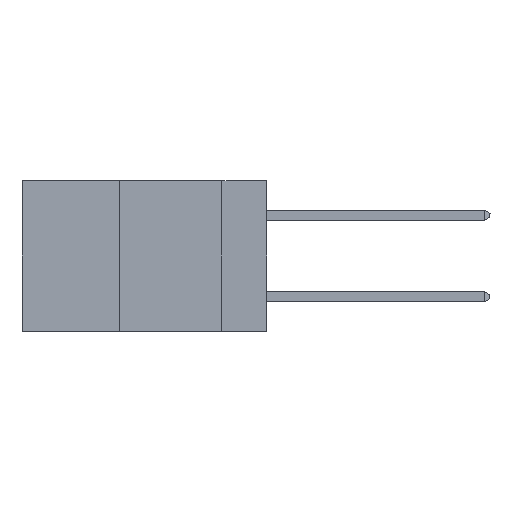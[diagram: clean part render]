
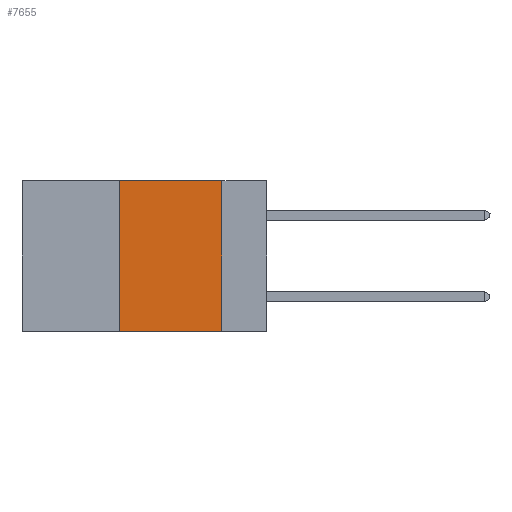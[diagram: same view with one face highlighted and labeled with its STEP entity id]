
A CAD part, left-side view. The second image highlights one B-rep face of the part: STEP entity #7655.
In plain terms, the highlighted planar face has unit normal (-1, 0, 0).
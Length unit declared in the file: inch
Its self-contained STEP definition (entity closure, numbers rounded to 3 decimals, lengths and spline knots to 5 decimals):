
#302 = LINE ( 'NONE', #19538, #10759 ) ;
#681 = PLANE ( 'NONE',  #7395 ) ;
#1203 = EDGE_CURVE ( 'NONE', #21719, #1650, #18108, .T. ) ;
#1267 = CARTESIAN_POINT ( 'NONE',  ( 0., 0.6, -0.37 ) ) ;
#1316 = VECTOR ( 'NONE', #17362, 39.37008 ) ;
#1650 = VERTEX_POINT ( 'NONE', #8465 ) ;
#2507 = DIRECTION ( 'NONE',  ( 1., 0., 0. ) ) ;
#2869 = DIRECTION ( 'NONE',  ( 0., -1., 0. ) ) ;
#3205 = LINE ( 'NONE', #1267, #8802 ) ;
#4940 = VECTOR ( 'NONE', #6041, 39.37008 ) ;
#5548 = DIRECTION ( 'NONE',  ( 0., 0., 1. ) ) ;
#6041 = DIRECTION ( 'NONE',  ( 0., 0., -1. ) ) ;
#6536 = EDGE_CURVE ( 'NONE', #13999, #1650, #3205, .T. ) ;
#6560 = ORIENTED_EDGE ( 'NONE', *, *, #6536, .T. ) ;
#6569 = ORIENTED_EDGE ( 'NONE', *, *, #14269, .F. ) ;
#7348 = CARTESIAN_POINT ( 'NONE',  ( 0., 0.11, 0. ) ) ;
#7395 = AXIS2_PLACEMENT_3D ( 'NONE', #21307, #2507, #7962 ) ;
#7655 = ADVANCED_FACE ( 'NONE', ( #18112 ), #681, .F. ) ;
#7962 = DIRECTION ( 'NONE',  ( 0., 0., -1. ) ) ;
#8093 = ORIENTED_EDGE ( 'NONE', *, *, #1203, .F. ) ;
#8243 = ORIENTED_EDGE ( 'NONE', *, *, #14006, .F. ) ;
#8465 = CARTESIAN_POINT ( 'NONE',  ( 0., 0.11, -0.37 ) ) ;
#8799 = CARTESIAN_POINT ( 'NONE',  ( 0., 0.6, 0. ) ) ;
#8802 = VECTOR ( 'NONE', #2869, 39.37008 ) ;
#9215 = CARTESIAN_POINT ( 'NONE',  ( 0., 0.11, 0. ) ) ;
#9506 = VERTEX_POINT ( 'NONE', #21395 ) ;
#10759 = VECTOR ( 'NONE', #5548, 39.37008 ) ;
#13999 = VERTEX_POINT ( 'NONE', #18053 ) ;
#14006 = EDGE_CURVE ( 'NONE', #13999, #9506, #302, .T. ) ;
#14269 = EDGE_CURVE ( 'NONE', #9506, #21719, #20765, .T. ) ;
#16131 = EDGE_LOOP ( 'NONE', ( #8093, #6569, #8243, #6560 ) ) ;
#17362 = DIRECTION ( 'NONE',  ( 0., -1., 0. ) ) ;
#18053 = CARTESIAN_POINT ( 'NONE',  ( 0., 0.36, -0.37 ) ) ;
#18108 = LINE ( 'NONE', #9215, #4940 ) ;
#18112 = FACE_OUTER_BOUND ( 'NONE', #16131, .T. ) ;
#19538 = CARTESIAN_POINT ( 'NONE',  ( 0., 0.36, 0. ) ) ;
#20765 = LINE ( 'NONE', #8799, #1316 ) ;
#21307 = CARTESIAN_POINT ( 'NONE',  ( 0., 0.6, 0. ) ) ;
#21395 = CARTESIAN_POINT ( 'NONE',  ( 0., 0.36, 0. ) ) ;
#21719 = VERTEX_POINT ( 'NONE', #7348 ) ;
